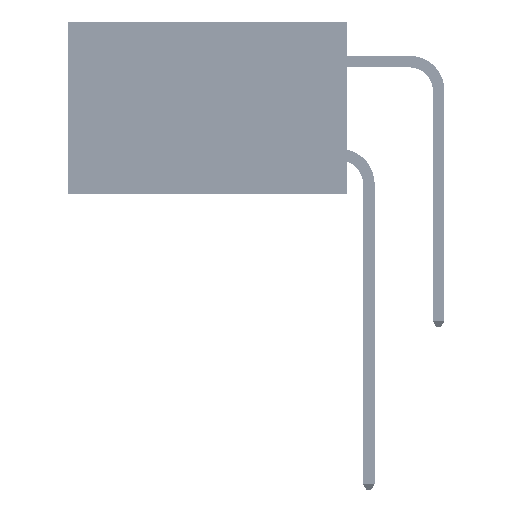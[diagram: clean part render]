
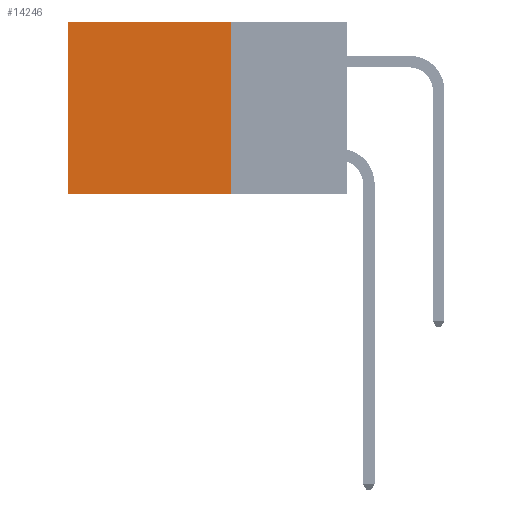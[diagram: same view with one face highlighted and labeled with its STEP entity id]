
A CAD part, left-side view. The second image highlights one B-rep face of the part: STEP entity #14246.
In plain terms, the highlighted planar face has unit normal (-1, 0, 0).
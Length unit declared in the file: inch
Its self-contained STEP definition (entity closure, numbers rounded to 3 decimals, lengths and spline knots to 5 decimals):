
#507 = CARTESIAN_POINT ( 'NONE',  ( 0.2875, 0.6, 0. ) ) ;
#839 = LINE ( 'NONE', #16869, #38708 ) ;
#2666 = DIRECTION ( 'NONE',  ( 1., 0., 0. ) ) ;
#4385 = CARTESIAN_POINT ( 'NONE',  ( 0.2875, 0.6, -0.37 ) ) ;
#4751 = EDGE_CURVE ( 'NONE', #5619, #32084, #839, .T. ) ;
#5475 = VERTEX_POINT ( 'NONE', #507 ) ;
#5560 = CARTESIAN_POINT ( 'NONE',  ( 0.2875, 0.25, 0. ) ) ;
#5619 = VERTEX_POINT ( 'NONE', #39101 ) ;
#8949 = EDGE_CURVE ( 'NONE', #5475, #14617, #44761, .T. ) ;
#9071 = AXIS2_PLACEMENT_3D ( 'NONE', #21131, #2666, #10188 ) ;
#9342 = CARTESIAN_POINT ( 'NONE',  ( 0.2875, 0.25, -0.37 ) ) ;
#9852 = LINE ( 'NONE', #20781, #23052 ) ;
#10188 = DIRECTION ( 'NONE',  ( 0., 0., -1. ) ) ;
#10445 = ORIENTED_EDGE ( 'NONE', *, *, #4751, .F. ) ;
#13045 = DIRECTION ( 'NONE',  ( 0., 1., 0. ) ) ;
#14246 = ADVANCED_FACE ( 'NONE', ( #34718 ), #46953, .F. ) ;
#14617 = VERTEX_POINT ( 'NONE', #4385 ) ;
#16869 = CARTESIAN_POINT ( 'NONE',  ( 0.2875, 0.25, 0. ) ) ;
#18377 = EDGE_CURVE ( 'NONE', #5619, #5475, #29081, .T. ) ;
#20781 = CARTESIAN_POINT ( 'NONE',  ( 0.2875, 0.25, -0.37 ) ) ;
#21131 = CARTESIAN_POINT ( 'NONE',  ( 0.2875, 0.25, 0. ) ) ;
#22095 = DIRECTION ( 'NONE',  ( 0., 0., -1. ) ) ;
#22429 = CARTESIAN_POINT ( 'NONE',  ( 0.2875, 0.6, 0. ) ) ;
#23052 = VECTOR ( 'NONE', #13045, 39.37008 ) ;
#23305 = EDGE_CURVE ( 'NONE', #32084, #14617, #9852, .T. ) ;
#25997 = ORIENTED_EDGE ( 'NONE', *, *, #23305, .F. ) ;
#28067 = VECTOR ( 'NONE', #22095, 39.37008 ) ;
#29081 = LINE ( 'NONE', #5560, #31380 ) ;
#31380 = VECTOR ( 'NONE', #45716, 39.37008 ) ;
#31579 = DIRECTION ( 'NONE',  ( 0., 0., -1. ) ) ;
#32084 = VERTEX_POINT ( 'NONE', #9342 ) ;
#34718 = FACE_OUTER_BOUND ( 'NONE', #47096, .T. ) ;
#36963 = ORIENTED_EDGE ( 'NONE', *, *, #8949, .T. ) ;
#38708 = VECTOR ( 'NONE', #31579, 39.37008 ) ;
#39101 = CARTESIAN_POINT ( 'NONE',  ( 0.2875, 0.25, 0. ) ) ;
#44761 = LINE ( 'NONE', #22429, #28067 ) ;
#45716 = DIRECTION ( 'NONE',  ( 0., 1., 0. ) ) ;
#46315 = ORIENTED_EDGE ( 'NONE', *, *, #18377, .T. ) ;
#46953 = PLANE ( 'NONE',  #9071 ) ;
#47096 = EDGE_LOOP ( 'NONE', ( #36963, #25997, #10445, #46315 ) ) ;
